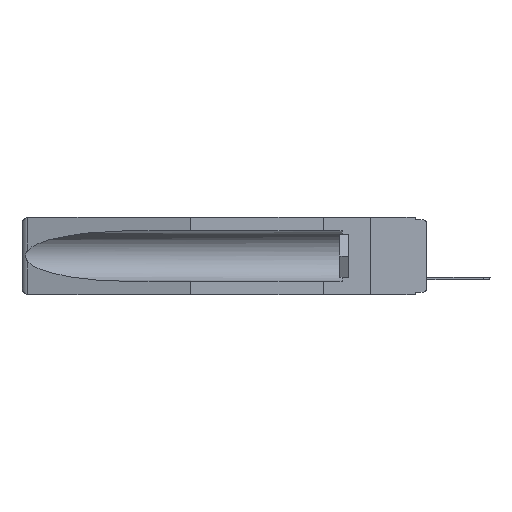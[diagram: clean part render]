
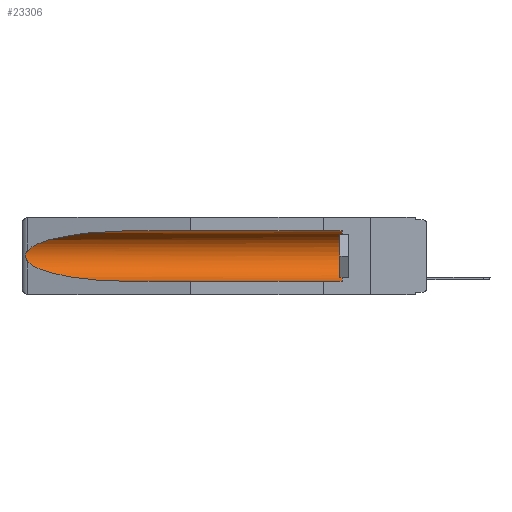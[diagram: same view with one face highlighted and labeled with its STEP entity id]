
A CAD part, left-side view. The second image highlights one B-rep face of the part: STEP entity #23306.
In plain terms, the highlighted cylindrical face has radius 2.857 mm (diameter 5.715 mm), a partial arc.
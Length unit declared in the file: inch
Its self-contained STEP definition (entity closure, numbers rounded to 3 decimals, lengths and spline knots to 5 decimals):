
#345 = EDGE_CURVE ( 'NONE', #6214, #10176, #19486, .T. ) ;
#659 = CARTESIAN_POINT ( 'NONE',  ( 0.2675, 1.53308, -0.16763 ) ) ;
#1239 = EDGE_CURVE ( 'NONE', #10176, #7555, #11596, .T. ) ;
#1580 = CARTESIAN_POINT ( 'NONE',  ( 0.26537, 1.52718, -0.14972 ) ) ;
#1842 = CARTESIAN_POINT ( 'NONE',  ( 0.25451, 1.48313, -0.24835 ) ) ;
#2038 = ORIENTED_EDGE ( 'NONE', *, *, #2513, .T. ) ;
#2513 = EDGE_CURVE ( 'NONE', #17426, #3926, #13336, .T. ) ;
#2534 = CARTESIAN_POINT ( 'NONE',  ( 0.26597, 1.5296, -0.19026 ) ) ;
#2771 = CARTESIAN_POINT ( 'NONE',  ( 0.26654, 1.53092, -0.15636 ) ) ;
#2880 = VECTOR ( 'NONE', #17918, 39.37008 ) ;
#3445 = CARTESIAN_POINT ( 'NONE',  ( 0.155, 1.07973, -0.059 ) ) ;
#3926 = VERTEX_POINT ( 'NONE', #12136 ) ;
#4014 = CARTESIAN_POINT ( 'NONE',  ( 0.155, -0.30754, -0.1715 ) ) ;
#4015 = VERTEX_POINT ( 'NONE', #6075 ) ;
#5174 = FACE_OUTER_BOUND ( 'NONE', #11333, .T. ) ;
#5825 = CARTESIAN_POINT ( 'NONE',  ( 0.155, 1.07973, -0.284 ) ) ;
#6075 = CARTESIAN_POINT ( 'NONE',  ( 0.155, 0.126, -0.284 ) ) ;
#6205 = CARTESIAN_POINT ( 'NONE',  ( 0.155, 0.126, -0.1715 ) ) ;
#6214 = VERTEX_POINT ( 'NONE', #16821 ) ;
#7329 = CARTESIAN_POINT ( 'NONE',  ( 0.26537, 1.52718, -0.19328 ) ) ;
#7540 = AXIS2_PLACEMENT_3D ( 'NONE', #6205, #22793, #10043 ) ;
#7555 = VERTEX_POINT ( 'NONE', #1580 ) ;
#8021 = AXIS2_PLACEMENT_3D ( 'NONE', #4014, #10898, #9029 ) ;
#9029 = DIRECTION ( 'NONE',  ( 0., 0., 1. ) ) ;
#10043 = DIRECTION ( 'NONE',  ( 0., 0., 1. ) ) ;
#10176 = VERTEX_POINT ( 'NONE', #21743 ) ;
#10306 = CIRCLE ( 'NONE', #7540, 0.1125 ) ;
#10347 = CARTESIAN_POINT ( 'NONE',  ( 0.2675, 1.53308, -0.17534 ) ) ;
#10898 = DIRECTION ( 'NONE',  ( 0., 1., 0. ) ) ;
#11333 = EDGE_LOOP ( 'NONE', ( #16222, #21691, #2038, #14735, #15775, #18406 ) ) ;
#11596 =( BOUNDED_CURVE ( )  B_SPLINE_CURVE ( 3, ( #3445, #24013, #18698, #18934 ),
 .UNSPECIFIED., .F., .F. ) 
 B_SPLINE_CURVE_WITH_KNOTS ( ( 4, 4 ),
 ( 4.71239, 6.08839 ),
 .UNSPECIFIED. ) 
 CURVE ( )  GEOMETRIC_REPRESENTATION_ITEM ( )  RATIONAL_B_SPLINE_CURVE ( ( 1., 0.848, 0.848, 1. ) ) 
 REPRESENTATION_ITEM ( '' )  );
#12136 = CARTESIAN_POINT ( 'NONE',  ( 0.155, 1.07973, -0.284 ) ) ;
#12395 = EDGE_CURVE ( 'NONE', #4015, #6214, #10306, .T. ) ;
#13336 =( BOUNDED_CURVE ( )  B_SPLINE_CURVE ( 3, ( #7329, #1842, #18816, #5825 ),
 .UNSPECIFIED., .F., .F. ) 
 B_SPLINE_CURVE_WITH_KNOTS ( ( 4, 4 ),
 ( 0.1948, 1.5708 ),
 .UNSPECIFIED. ) 
 CURVE ( )  GEOMETRIC_REPRESENTATION_ITEM ( )  RATIONAL_B_SPLINE_CURVE ( ( 1., 0.848, 0.848, 1. ) ) 
 REPRESENTATION_ITEM ( '' )  );
#13581 = CARTESIAN_POINT ( 'NONE',  ( 0.26537, 1.52718, -0.19328 ) ) ;
#13584 = CYLINDRICAL_SURFACE ( 'NONE', #8021, 0.1125 ) ;
#13826 = CARTESIAN_POINT ( 'NONE',  ( 0.26537, 1.52718, -0.14972 ) ) ;
#13929 = B_SPLINE_CURVE_WITH_KNOTS ( 'NONE', 3,
 ( #13826, #21607, #2771, #14184, #659, #10347, #21230, #19628, #2534, #19508 ),
 .UNSPECIFIED., .F., .F.,
 ( 4, 2, 2, 2, 4 ),
 ( 0., 0.00029, 0.00058, 0.00087, 0.00117 ),
 .UNSPECIFIED. ) ;
#14164 = CARTESIAN_POINT ( 'NONE',  ( 0.155, -0.30754, -0.059 ) ) ;
#14184 = CARTESIAN_POINT ( 'NONE',  ( 0.2673, 1.5327, -0.16383 ) ) ;
#14735 = ORIENTED_EDGE ( 'NONE', *, *, #17099, .F. ) ;
#15775 = ORIENTED_EDGE ( 'NONE', *, *, #12395, .T. ) ;
#16024 = DIRECTION ( 'NONE',  ( 0., 1., 0. ) ) ;
#16222 = ORIENTED_EDGE ( 'NONE', *, *, #1239, .T. ) ;
#16821 = CARTESIAN_POINT ( 'NONE',  ( 0.155, 0.126, -0.059 ) ) ;
#17099 = EDGE_CURVE ( 'NONE', #4015, #3926, #23244, .T. ) ;
#17426 = VERTEX_POINT ( 'NONE', #13581 ) ;
#17797 = CARTESIAN_POINT ( 'NONE',  ( 0.155, -0.30754, -0.284 ) ) ;
#17918 = DIRECTION ( 'NONE',  ( 0., 1., 0. ) ) ;
#18406 = ORIENTED_EDGE ( 'NONE', *, *, #345, .T. ) ;
#18698 = CARTESIAN_POINT ( 'NONE',  ( 0.25451, 1.48313, -0.09465 ) ) ;
#18816 = CARTESIAN_POINT ( 'NONE',  ( 0.21114, 1.30732, -0.284 ) ) ;
#18934 = CARTESIAN_POINT ( 'NONE',  ( 0.26537, 1.52718, -0.14972 ) ) ;
#19486 = LINE ( 'NONE', #14164, #20060 ) ;
#19508 = CARTESIAN_POINT ( 'NONE',  ( 0.26537, 1.52718, -0.19328 ) ) ;
#19628 = CARTESIAN_POINT ( 'NONE',  ( 0.26655, 1.53094, -0.18657 ) ) ;
#20060 = VECTOR ( 'NONE', #16024, 39.37008 ) ;
#21230 = CARTESIAN_POINT ( 'NONE',  ( 0.2673, 1.53269, -0.17917 ) ) ;
#21607 = CARTESIAN_POINT ( 'NONE',  ( 0.26597, 1.52961, -0.15275 ) ) ;
#21691 = ORIENTED_EDGE ( 'NONE', *, *, #23429, .T. ) ;
#21743 = CARTESIAN_POINT ( 'NONE',  ( 0.155, 1.07973, -0.059 ) ) ;
#22793 = DIRECTION ( 'NONE',  ( 0., -1., 0. ) ) ;
#23244 = LINE ( 'NONE', #17797, #2880 ) ;
#23306 = ADVANCED_FACE ( 'NONE', ( #5174 ), #13584, .F. ) ;
#23429 = EDGE_CURVE ( 'NONE', #7555, #17426, #13929, .T. ) ;
#24013 = CARTESIAN_POINT ( 'NONE',  ( 0.21114, 1.30732, -0.059 ) ) ;
